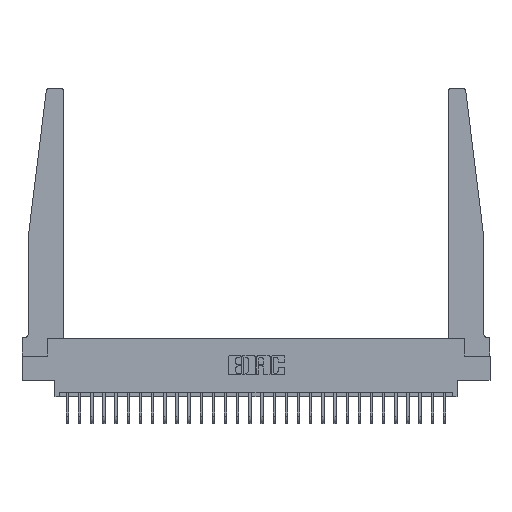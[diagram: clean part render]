
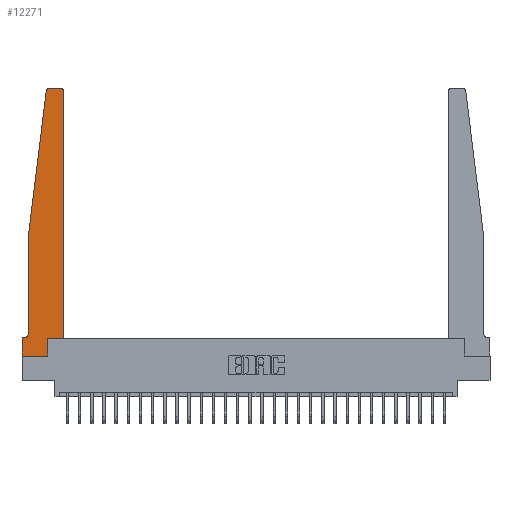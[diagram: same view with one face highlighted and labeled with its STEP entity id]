
A CAD part, top view. The second image highlights one B-rep face of the part: STEP entity #12271.
In plain terms, the highlighted planar face has unit normal (0, 0, 1).
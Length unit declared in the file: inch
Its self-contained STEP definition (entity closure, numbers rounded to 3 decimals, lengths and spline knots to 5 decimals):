
#74 = CARTESIAN_POINT ( 'NONE',  ( 0., 0., 0.37 ) ) ;
#246 = EDGE_LOOP ( 'NONE', ( #2975, #9937, #24028, #18857, #19435, #22635, #7300, #26856, #22886, #19156, #23515, #28764 ) ) ;
#987 = CIRCLE ( 'NONE', #10003, 0.03 ) ;
#1968 = EDGE_CURVE ( 'NONE', #15286, #20723, #18480, .T. ) ;
#2975 = ORIENTED_EDGE ( 'NONE', *, *, #17678, .T. ) ;
#3227 = CARTESIAN_POINT ( 'NONE',  ( 0.425, 0.18, 0.37 ) ) ;
#3329 = CARTESIAN_POINT ( 'NONE',  ( 0.395, 2.75, 0.37 ) ) ;
#3363 = LINE ( 'NONE', #24285, #12104 ) ;
#4592 = CARTESIAN_POINT ( 'NONE',  ( 0.27653, 2.75, 0.37 ) ) ;
#4666 = EDGE_CURVE ( 'NONE', #25125, #11964, #15589, .T. ) ;
#4773 = EDGE_CURVE ( 'NONE', #5335, #24752, #4890, .T. ) ;
#4890 = LINE ( 'NONE', #11883, #5185 ) ;
#5185 = VECTOR ( 'NONE', #7136, 39.37008 ) ;
#5335 = VERTEX_POINT ( 'NONE', #3227 ) ;
#6028 = DIRECTION ( 'NONE',  ( 1., 0., 0. ) ) ;
#6735 = CARTESIAN_POINT ( 'NONE',  ( 0.2605, 0.18, 0.37 ) ) ;
#6741 = VERTEX_POINT ( 'NONE', #74 ) ;
#7035 = LINE ( 'NONE', #14011, #14517 ) ;
#7136 = DIRECTION ( 'NONE',  ( 0., 1., 0. ) ) ;
#7300 = ORIENTED_EDGE ( 'NONE', *, *, #9123, .T. ) ;
#8006 = DIRECTION ( 'NONE',  ( 0., -1., 0. ) ) ;
#8570 = EDGE_CURVE ( 'NONE', #11964, #19034, #7035, .T. ) ;
#8699 = DIRECTION ( 'NONE',  ( 0., 0., 1. ) ) ;
#8780 = CARTESIAN_POINT ( 'NONE',  ( 0.425, 0.18, 0.37 ) ) ;
#9123 = EDGE_CURVE ( 'NONE', #20723, #6741, #14832, .T. ) ;
#9858 = FACE_OUTER_BOUND ( 'NONE', #246, .T. ) ;
#9919 = AXIS2_PLACEMENT_3D ( 'NONE', #20022, #8699, #13015 ) ;
#9937 = ORIENTED_EDGE ( 'NONE', *, *, #21376, .T. ) ;
#10003 = AXIS2_PLACEMENT_3D ( 'NONE', #24496, #16023, #22266 ) ;
#10505 = DIRECTION ( 'NONE',  ( -1., 0., 0. ) ) ;
#11555 = AXIS2_PLACEMENT_3D ( 'NONE', #25911, #23809, #27996 ) ;
#11883 = CARTESIAN_POINT ( 'NONE',  ( 0.425, 0.18, 0.37 ) ) ;
#11964 = VERTEX_POINT ( 'NONE', #17918 ) ;
#12104 = VECTOR ( 'NONE', #6028, 39.37008 ) ;
#12263 = CARTESIAN_POINT ( 'NONE',  ( 0.2605, 0.18, 0.37 ) ) ;
#12271 = ADVANCED_FACE ( 'NONE', ( #9858 ), #18936, .T. ) ;
#12287 = VECTOR ( 'NONE', #10505, 39.37008 ) ;
#12678 = CARTESIAN_POINT ( 'NONE',  ( 0.015, 0.1875, 0.37 ) ) ;
#12917 = DIRECTION ( 'NONE',  ( -0.122, -0.992, 0. ) ) ;
#13015 = DIRECTION ( 'NONE',  ( 1., 0., 0. ) ) ;
#13422 = VECTOR ( 'NONE', #24843, 39.37008 ) ;
#14011 = CARTESIAN_POINT ( 'NONE',  ( 0.065, 1.25, 0.37 ) ) ;
#14182 = DIRECTION ( 'NONE',  ( 0., 0., -1. ) ) ;
#14517 = VECTOR ( 'NONE', #22640, 39.37008 ) ;
#14643 = DIRECTION ( 'NONE',  ( 0., 1., 0. ) ) ;
#14669 = CARTESIAN_POINT ( 'NONE',  ( 0.25, 2.75, 0.37 ) ) ;
#14763 = CARTESIAN_POINT ( 'NONE',  ( 0.065, 0.2375, 0.37 ) ) ;
#14832 = LINE ( 'NONE', #19023, #21234 ) ;
#15286 = VERTEX_POINT ( 'NONE', #12678 ) ;
#15304 = CARTESIAN_POINT ( 'NONE',  ( 0., 0.1875, 0.37 ) ) ;
#15485 = VERTEX_POINT ( 'NONE', #6735 ) ;
#15589 = LINE ( 'NONE', #28843, #28924 ) ;
#16023 = DIRECTION ( 'NONE',  ( 0., 0., 1. ) ) ;
#16279 = CARTESIAN_POINT ( 'NONE',  ( 0.2605, 0., 0.37 ) ) ;
#16405 = VERTEX_POINT ( 'NONE', #16279 ) ;
#16705 = DIRECTION ( 'NONE',  ( -1., 0., 0. ) ) ;
#16731 = VECTOR ( 'NONE', #18018, 39.37008 ) ;
#17041 = CARTESIAN_POINT ( 'NONE',  ( 0.24675, 2.72367, 0.37 ) ) ;
#17434 = LINE ( 'NONE', #8780, #16731 ) ;
#17678 = EDGE_CURVE ( 'NONE', #29073, #24454, #28356, .T. ) ;
#17880 = EDGE_CURVE ( 'NONE', #24752, #29073, #22734, .T. ) ;
#17918 = CARTESIAN_POINT ( 'NONE',  ( 0.065, 1.25, 0.37 ) ) ;
#18018 = DIRECTION ( 'NONE',  ( 1., 0., 0. ) ) ;
#18480 = LINE ( 'NONE', #22633, #13422 ) ;
#18857 = ORIENTED_EDGE ( 'NONE', *, *, #8570, .T. ) ;
#18936 = PLANE ( 'NONE',  #11555 ) ;
#19023 = CARTESIAN_POINT ( 'NONE',  ( 0., 0., 0.37 ) ) ;
#19034 = VERTEX_POINT ( 'NONE', #14763 ) ;
#19079 = CARTESIAN_POINT ( 'NONE',  ( 0.015, 0.2375, 0.37 ) ) ;
#19156 = ORIENTED_EDGE ( 'NONE', *, *, #23869, .T. ) ;
#19435 = ORIENTED_EDGE ( 'NONE', *, *, #26808, .T. ) ;
#20022 = CARTESIAN_POINT ( 'NONE',  ( 0.395, 2.72, 0.37 ) ) ;
#20723 = VERTEX_POINT ( 'NONE', #15304 ) ;
#21234 = VECTOR ( 'NONE', #8006, 39.37008 ) ;
#21376 = EDGE_CURVE ( 'NONE', #24454, #25125, #987, .T. ) ;
#22096 = CARTESIAN_POINT ( 'NONE',  ( 0.425, 2.72, 0.37 ) ) ;
#22266 = DIRECTION ( 'NONE',  ( 1., 0., 0. ) ) ;
#22633 = CARTESIAN_POINT ( 'NONE',  ( 0.065, 0.1875, 0.37 ) ) ;
#22635 = ORIENTED_EDGE ( 'NONE', *, *, #1968, .T. ) ;
#22640 = DIRECTION ( 'NONE',  ( 0., -1., 0. ) ) ;
#22734 = CIRCLE ( 'NONE', #9919, 0.03 ) ;
#22886 = ORIENTED_EDGE ( 'NONE', *, *, #25096, .T. ) ;
#23515 = ORIENTED_EDGE ( 'NONE', *, *, #4773, .T. ) ;
#23809 = DIRECTION ( 'NONE',  ( 0., 0., 1. ) ) ;
#23869 = EDGE_CURVE ( 'NONE', #15485, #5335, #17434, .T. ) ;
#23901 = CIRCLE ( 'NONE', #23975, 0.05 ) ;
#23903 = VECTOR ( 'NONE', #14643, 39.37008 ) ;
#23975 = AXIS2_PLACEMENT_3D ( 'NONE', #19079, #14182, #16705 ) ;
#24028 = ORIENTED_EDGE ( 'NONE', *, *, #4666, .T. ) ;
#24285 = CARTESIAN_POINT ( 'NONE',  ( 0., 0., 0.37 ) ) ;
#24454 = VERTEX_POINT ( 'NONE', #4592 ) ;
#24496 = CARTESIAN_POINT ( 'NONE',  ( 0.27653, 2.72, 0.37 ) ) ;
#24752 = VERTEX_POINT ( 'NONE', #22096 ) ;
#24843 = DIRECTION ( 'NONE',  ( -1., 0., 0. ) ) ;
#25096 = EDGE_CURVE ( 'NONE', #16405, #15485, #28327, .T. ) ;
#25125 = VERTEX_POINT ( 'NONE', #17041 ) ;
#25911 = CARTESIAN_POINT ( 'NONE',  ( 0., 0.1875, 0.37 ) ) ;
#26808 = EDGE_CURVE ( 'NONE', #19034, #15286, #23901, .T. ) ;
#26856 = ORIENTED_EDGE ( 'NONE', *, *, #28563, .T. ) ;
#27996 = DIRECTION ( 'NONE',  ( 1., 0., 0. ) ) ;
#28327 = LINE ( 'NONE', #12263, #23903 ) ;
#28356 = LINE ( 'NONE', #14669, #12287 ) ;
#28563 = EDGE_CURVE ( 'NONE', #6741, #16405, #3363, .T. ) ;
#28764 = ORIENTED_EDGE ( 'NONE', *, *, #17880, .T. ) ;
#28843 = CARTESIAN_POINT ( 'NONE',  ( 0.065, 1.25, 0.37 ) ) ;
#28924 = VECTOR ( 'NONE', #12917, 39.37008 ) ;
#29073 = VERTEX_POINT ( 'NONE', #3329 ) ;
